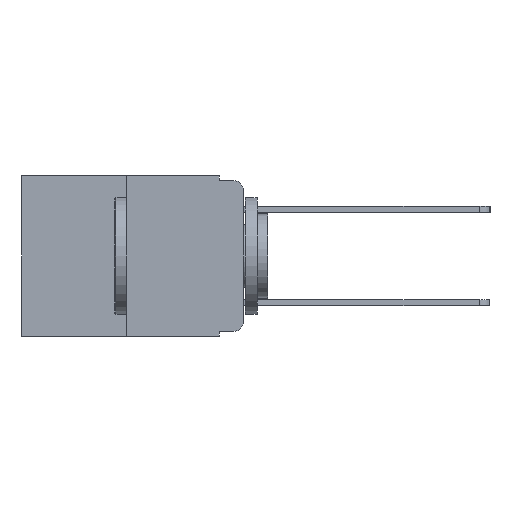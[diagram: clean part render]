
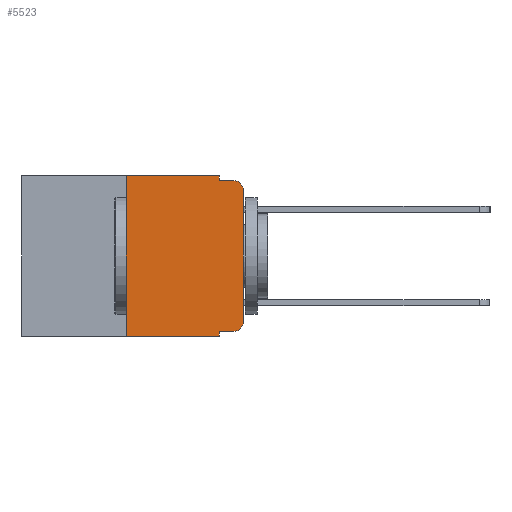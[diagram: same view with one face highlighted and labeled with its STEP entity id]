
A CAD part, left-side view. The second image highlights one B-rep face of the part: STEP entity #5523.
In plain terms, the highlighted planar face has unit normal (-1, 0, 0).
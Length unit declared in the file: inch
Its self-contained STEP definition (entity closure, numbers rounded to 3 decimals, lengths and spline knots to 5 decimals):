
#1130 = VECTOR ( 'NONE', #5022, 39.37008 ) ;
#1148 = ORIENTED_EDGE ( 'NONE', *, *, #1337, .T. ) ;
#1198 = VECTOR ( 'NONE', #6045, 39.37008 ) ;
#1223 = CARTESIAN_POINT ( 'NONE',  ( 0., 0.02, -0.01 ) ) ;
#1248 = AXIS2_PLACEMENT_3D ( 'NONE', #11161, #11155, #11131 ) ;
#1337 = EDGE_CURVE ( 'NONE', #1691, #9869, #4030, .T. ) ;
#1344 = ORIENTED_EDGE ( 'NONE', *, *, #2428, .T. ) ;
#1456 = LINE ( 'NONE', #8116, #8877 ) ;
#1573 = ORIENTED_EDGE ( 'NONE', *, *, #4509, .F. ) ;
#1691 = VERTEX_POINT ( 'NONE', #6633 ) ;
#1799 = CARTESIAN_POINT ( 'NONE',  ( 0., 0.051, -0.01 ) ) ;
#1866 = LINE ( 'NONE', #7053, #9479 ) ;
#1930 = VERTEX_POINT ( 'NONE', #12111 ) ;
#2199 = VERTEX_POINT ( 'NONE', #6304 ) ;
#2428 = EDGE_CURVE ( 'NONE', #1930, #5693, #8933, .T. ) ;
#2513 = DIRECTION ( 'NONE',  ( -1., 0., 0. ) ) ;
#2529 = CARTESIAN_POINT ( 'NONE',  ( 0., 0.051, -0.343 ) ) ;
#2770 = AXIS2_PLACEMENT_3D ( 'NONE', #8549, #2513, #9416 ) ;
#3136 = EDGE_CURVE ( 'NONE', #5857, #1930, #7636, .T. ) ;
#3213 = DIRECTION ( 'NONE',  ( 0., 0., -1. ) ) ;
#3228 = ORIENTED_EDGE ( 'NONE', *, *, #6546, .F. ) ;
#3335 = ORIENTED_EDGE ( 'NONE', *, *, #5176, .F. ) ;
#3484 = ORIENTED_EDGE ( 'NONE', *, *, #7247, .T. ) ;
#3949 = ORIENTED_EDGE ( 'NONE', *, *, #7896, .T. ) ;
#4030 = LINE ( 'NONE', #9085, #1198 ) ;
#4398 = DIRECTION ( 'NONE',  ( 0., 0., 1. ) ) ;
#4509 = EDGE_CURVE ( 'NONE', #5857, #9869, #11502, .T. ) ;
#4712 = DIRECTION ( 'NONE',  ( 1., 0., 0. ) ) ;
#4746 = LINE ( 'NONE', #9342, #11903 ) ;
#4863 = CARTESIAN_POINT ( 'NONE',  ( 0., 0.051, 0. ) ) ;
#4940 = DIRECTION ( 'NONE',  ( 0., -1., 0. ) ) ;
#4960 = ORIENTED_EDGE ( 'NONE', *, *, #11088, .F. ) ;
#4963 = CARTESIAN_POINT ( 'NONE',  ( 0., 0.051, 0. ) ) ;
#5022 = DIRECTION ( 'NONE',  ( 0., 0., -1. ) ) ;
#5041 = FACE_OUTER_BOUND ( 'NONE', #7381, .T. ) ;
#5176 = EDGE_CURVE ( 'NONE', #1691, #12482, #4746, .T. ) ;
#5523 = ADVANCED_FACE ( 'NONE', ( #5041 ), #9524, .F. ) ;
#5693 = VERTEX_POINT ( 'NONE', #10356 ) ;
#5857 = VERTEX_POINT ( 'NONE', #10591 ) ;
#5860 = EDGE_CURVE ( 'NONE', #8509, #2199, #1456, .T. ) ;
#6045 = DIRECTION ( 'NONE',  ( 0., -1., 0. ) ) ;
#6304 = CARTESIAN_POINT ( 'NONE',  ( 0., 0.051, -0.01 ) ) ;
#6426 = VECTOR ( 'NONE', #4940, 39.37008 ) ;
#6546 = EDGE_CURVE ( 'NONE', #2199, #11355, #8972, .T. ) ;
#6633 = CARTESIAN_POINT ( 'NONE',  ( 0., 0.25, -0.343 ) ) ;
#6770 = DIRECTION ( 'NONE',  ( 0., 0., 1. ) ) ;
#7053 = CARTESIAN_POINT ( 'NONE',  ( 0., 0.473, 0. ) ) ;
#7089 = CARTESIAN_POINT ( 'NONE',  ( 0., 0., -0.03 ) ) ;
#7247 = EDGE_CURVE ( 'NONE', #7525, #11355, #11408, .T. ) ;
#7335 = VECTOR ( 'NONE', #11906, 39.37008 ) ;
#7381 = EDGE_LOOP ( 'NONE', ( #3949, #3484, #3228, #8136, #4960, #3335, #1148, #1573, #10766, #1344 ) ) ;
#7525 = VERTEX_POINT ( 'NONE', #7089 ) ;
#7636 = LINE ( 'NONE', #9726, #7335 ) ;
#7896 = EDGE_CURVE ( 'NONE', #5693, #7525, #11255, .T. ) ;
#8031 = DIRECTION ( 'NONE',  ( 0., -1., 0. ) ) ;
#8116 = CARTESIAN_POINT ( 'NONE',  ( 0., 0.051, 0. ) ) ;
#8136 = ORIENTED_EDGE ( 'NONE', *, *, #5860, .F. ) ;
#8509 = VERTEX_POINT ( 'NONE', #4963 ) ;
#8549 = CARTESIAN_POINT ( 'NONE',  ( 0., 0.02, -0.03 ) ) ;
#8877 = VECTOR ( 'NONE', #3213, 39.37008 ) ;
#8933 = CIRCLE ( 'NONE', #1248, 0.02 ) ;
#8972 = LINE ( 'NONE', #1799, #6426 ) ;
#9085 = CARTESIAN_POINT ( 'NONE',  ( 0., 0.473, -0.343 ) ) ;
#9336 = AXIS2_PLACEMENT_3D ( 'NONE', #11045, #4712, #11286 ) ;
#9342 = CARTESIAN_POINT ( 'NONE',  ( 0., 0.25, 0. ) ) ;
#9393 = CARTESIAN_POINT ( 'NONE',  ( 0., 0.25, 0. ) ) ;
#9416 = DIRECTION ( 'NONE',  ( 0., 0., -1. ) ) ;
#9479 = VECTOR ( 'NONE', #8031, 39.37008 ) ;
#9524 = PLANE ( 'NONE',  #9336 ) ;
#9726 = CARTESIAN_POINT ( 'NONE',  ( 0., 0.051, -0.333 ) ) ;
#9869 = VERTEX_POINT ( 'NONE', #2529 ) ;
#10356 = CARTESIAN_POINT ( 'NONE',  ( 0., 0., -0.313 ) ) ;
#10591 = CARTESIAN_POINT ( 'NONE',  ( 0., 0.051, -0.333 ) ) ;
#10766 = ORIENTED_EDGE ( 'NONE', *, *, #3136, .T. ) ;
#10990 = VECTOR ( 'NONE', #6770, 39.37008 ) ;
#11045 = CARTESIAN_POINT ( 'NONE',  ( 0., 0.473, 0. ) ) ;
#11088 = EDGE_CURVE ( 'NONE', #12482, #8509, #1866, .T. ) ;
#11131 = DIRECTION ( 'NONE',  ( 0., 0., -1. ) ) ;
#11155 = DIRECTION ( 'NONE',  ( -1., 0., 0. ) ) ;
#11161 = CARTESIAN_POINT ( 'NONE',  ( 0., 0.02, -0.313 ) ) ;
#11255 = LINE ( 'NONE', #11613, #10990 ) ;
#11286 = DIRECTION ( 'NONE',  ( 0., 0., -1. ) ) ;
#11355 = VERTEX_POINT ( 'NONE', #1223 ) ;
#11408 = CIRCLE ( 'NONE', #2770, 0.02 ) ;
#11502 = LINE ( 'NONE', #4863, #1130 ) ;
#11613 = CARTESIAN_POINT ( 'NONE',  ( 0., 0., 0. ) ) ;
#11903 = VECTOR ( 'NONE', #4398, 39.37008 ) ;
#11906 = DIRECTION ( 'NONE',  ( 0., -1., 0. ) ) ;
#12111 = CARTESIAN_POINT ( 'NONE',  ( 0., 0.02, -0.333 ) ) ;
#12482 = VERTEX_POINT ( 'NONE', #9393 ) ;
